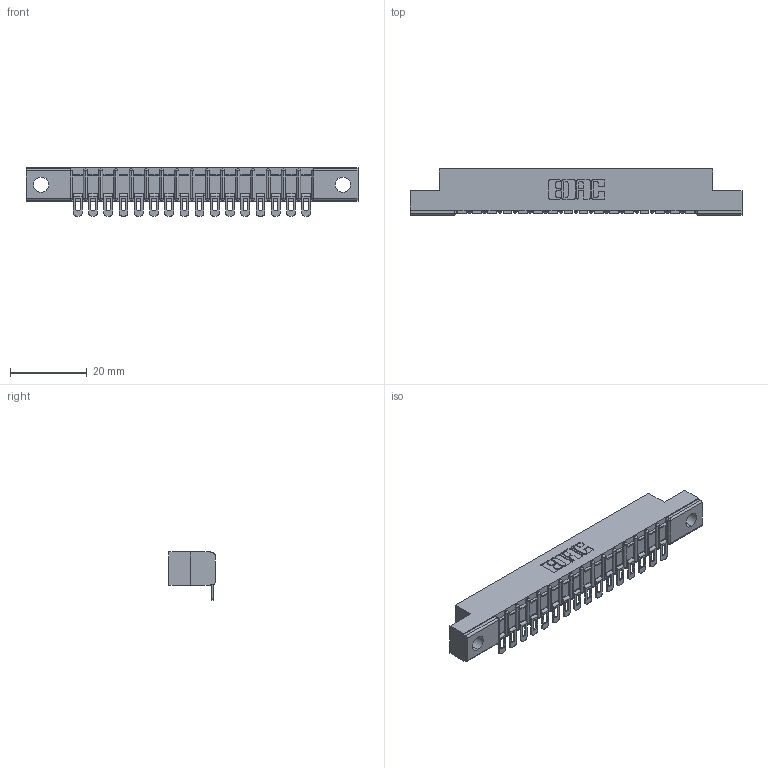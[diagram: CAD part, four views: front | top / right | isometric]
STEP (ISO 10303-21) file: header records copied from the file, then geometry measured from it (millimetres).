
FILE_DESCRIPTION (( 'STEP AP203' ), '1' );
FILE_NAME ('307-016-554-104.STEP', '2018-08-03T03:30:38', ( '' ), ( '' ), 'SwSTEP 2.0', 'SolidWorks 2016', '' );
FILE_SCHEMA (( 'CONFIG_CONTROL_DESIGN' ));
Length unit declared in the file: inch
Products named in the file (3): 307-016-554-104; 307 Part_.156 Dia Mounting Holes; 307-290-002_554
Assembly tree (17 placements, depth 2):
  307-016-554-104
    307 Part_.156 Dia Mounting Holes
    307-290-002_554  x16
Bounding box: 86.41 x 12.01 x 12.52 mm (x, y, z)
Volume: 5601.3 mm3; surface area: 9810.9 mm2
Topology: 17 solids, 17 shells, 1445 faces, 4407 edges, 2890 vertices
Faces by surface type: plane 820, cylinder 591, sphere 34
Entity records: 18305 total; most frequent: CARTESIAN_POINT 3088, ORIENTED_EDGE 3076, DIRECTION 3010, EDGE_CURVE 1538, LINE 1166, VECTOR 1166, VERTEX_POINT 1000, AXIS2_PLACEMENT_3D 922
